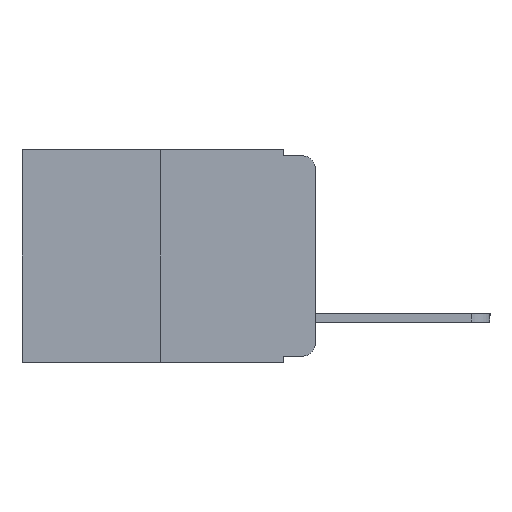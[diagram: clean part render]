
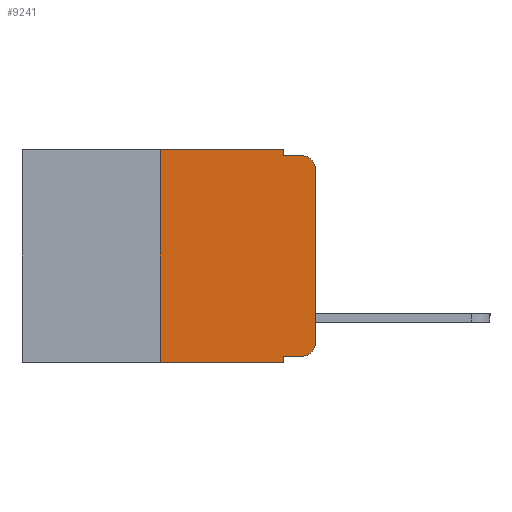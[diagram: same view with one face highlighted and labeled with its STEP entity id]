
A CAD part, left-side view. The second image highlights one B-rep face of the part: STEP entity #9241.
In plain terms, the highlighted planar face has unit normal (-1, 0, 0).
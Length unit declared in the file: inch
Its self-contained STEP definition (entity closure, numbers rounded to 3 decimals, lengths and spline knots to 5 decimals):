
#262 = LINE ( 'NONE', #21663, #22019 ) ;
#477 = CARTESIAN_POINT ( 'NONE',  ( 0., 0., -0.313 ) ) ;
#1154 = DIRECTION ( 'NONE',  ( 0., -1., 0. ) ) ;
#1220 = ORIENTED_EDGE ( 'NONE', *, *, #9397, .T. ) ;
#1235 = AXIS2_PLACEMENT_3D ( 'NONE', #17541, #7391, #19065 ) ;
#1457 = LINE ( 'NONE', #2063, #2033 ) ;
#1526 = VECTOR ( 'NONE', #12954, 39.37008 ) ;
#2030 = VECTOR ( 'NONE', #1154, 39.37008 ) ;
#2033 = VECTOR ( 'NONE', #12986, 39.37008 ) ;
#2063 = CARTESIAN_POINT ( 'NONE',  ( 0., 0.473, -0.343 ) ) ;
#2291 = CARTESIAN_POINT ( 'NONE',  ( 0., 0.051, 0. ) ) ;
#2404 = ORIENTED_EDGE ( 'NONE', *, *, #4663, .F. ) ;
#2716 = LINE ( 'NONE', #5729, #1526 ) ;
#2755 = VERTEX_POINT ( 'NONE', #20034 ) ;
#2882 = CARTESIAN_POINT ( 'NONE',  ( 0., 0.051, -0.343 ) ) ;
#3092 = DIRECTION ( 'NONE',  ( 0., 0., -1. ) ) ;
#3281 = VERTEX_POINT ( 'NONE', #19433 ) ;
#3611 = ORIENTED_EDGE ( 'NONE', *, *, #22121, .F. ) ;
#3684 = DIRECTION ( 'NONE',  ( -1., 0., 0. ) ) ;
#4008 = CARTESIAN_POINT ( 'NONE',  ( 0., 0.051, -0.333 ) ) ;
#4189 = ORIENTED_EDGE ( 'NONE', *, *, #5977, .T. ) ;
#4587 = CARTESIAN_POINT ( 'NONE',  ( 0., 0.02, -0.01 ) ) ;
#4663 = EDGE_CURVE ( 'NONE', #3281, #2755, #6049, .T. ) ;
#5001 = VERTEX_POINT ( 'NONE', #4008 ) ;
#5729 = CARTESIAN_POINT ( 'NONE',  ( 0., 0.051, -0.01 ) ) ;
#5977 = EDGE_CURVE ( 'NONE', #5001, #19971, #21554, .T. ) ;
#6049 = LINE ( 'NONE', #2291, #13855 ) ;
#6156 = CIRCLE ( 'NONE', #13313, 0.02 ) ;
#6426 = EDGE_CURVE ( 'NONE', #16449, #3281, #11781, .T. ) ;
#6481 = VERTEX_POINT ( 'NONE', #22135 ) ;
#6624 = DIRECTION ( 'NONE',  ( 0., -1., 0. ) ) ;
#6761 = CARTESIAN_POINT ( 'NONE',  ( 0., 0., -0.03 ) ) ;
#6831 = ORIENTED_EDGE ( 'NONE', *, *, #13273, .F. ) ;
#6907 = VECTOR ( 'NONE', #7201, 39.37008 ) ;
#7201 = DIRECTION ( 'NONE',  ( 0., 0., 1. ) ) ;
#7292 = EDGE_CURVE ( 'NONE', #6481, #16449, #10400, .T. ) ;
#7391 = DIRECTION ( 'NONE',  ( -1., 0., 0. ) ) ;
#7416 = ORIENTED_EDGE ( 'NONE', *, *, #6426, .F. ) ;
#8373 = VERTEX_POINT ( 'NONE', #2882 ) ;
#8388 = AXIS2_PLACEMENT_3D ( 'NONE', #12613, #19031, #9230 ) ;
#9230 = DIRECTION ( 'NONE',  ( 0., 0., -1. ) ) ;
#9241 = ADVANCED_FACE ( 'NONE', ( #13411 ), #14336, .F. ) ;
#9324 = EDGE_CURVE ( 'NONE', #6481, #8373, #1457, .T. ) ;
#9397 = EDGE_CURVE ( 'NONE', #9412, #12617, #18382, .T. ) ;
#9412 = VERTEX_POINT ( 'NONE', #477 ) ;
#9821 = CARTESIAN_POINT ( 'NONE',  ( 0., 0., 0. ) ) ;
#10215 = DIRECTION ( 'NONE',  ( 0., 0., -1. ) ) ;
#10400 = LINE ( 'NONE', #18922, #6907 ) ;
#11599 = VERTEX_POINT ( 'NONE', #4587 ) ;
#11781 = LINE ( 'NONE', #21665, #2030 ) ;
#12135 = ORIENTED_EDGE ( 'NONE', *, *, #7292, .F. ) ;
#12613 = CARTESIAN_POINT ( 'NONE',  ( 0., 0.473, 0. ) ) ;
#12617 = VERTEX_POINT ( 'NONE', #6761 ) ;
#12687 = ORIENTED_EDGE ( 'NONE', *, *, #9324, .T. ) ;
#12754 = CIRCLE ( 'NONE', #1235, 0.02 ) ;
#12954 = DIRECTION ( 'NONE',  ( 0., -1., 0. ) ) ;
#12986 = DIRECTION ( 'NONE',  ( 0., -1., 0. ) ) ;
#13184 = EDGE_LOOP ( 'NONE', ( #1220, #19649, #6831, #2404, #7416, #12135, #12687, #3611, #4189, #14291 ) ) ;
#13273 = EDGE_CURVE ( 'NONE', #2755, #11599, #2716, .T. ) ;
#13313 = AXIS2_PLACEMENT_3D ( 'NONE', #14408, #3684, #15995 ) ;
#13411 = FACE_OUTER_BOUND ( 'NONE', #13184, .T. ) ;
#13413 = CARTESIAN_POINT ( 'NONE',  ( 0., 0.25, 0. ) ) ;
#13855 = VECTOR ( 'NONE', #10215, 39.37008 ) ;
#14291 = ORIENTED_EDGE ( 'NONE', *, *, #21303, .T. ) ;
#14336 = PLANE ( 'NONE',  #8388 ) ;
#14408 = CARTESIAN_POINT ( 'NONE',  ( 0., 0.02, -0.313 ) ) ;
#15995 = DIRECTION ( 'NONE',  ( 0., 0., -1. ) ) ;
#16449 = VERTEX_POINT ( 'NONE', #13413 ) ;
#16971 = VECTOR ( 'NONE', #6624, 39.37008 ) ;
#17033 = EDGE_CURVE ( 'NONE', #12617, #11599, #12754, .T. ) ;
#17072 = CARTESIAN_POINT ( 'NONE',  ( 0., 0.02, -0.333 ) ) ;
#17541 = CARTESIAN_POINT ( 'NONE',  ( 0., 0.02, -0.03 ) ) ;
#18382 = LINE ( 'NONE', #9821, #21996 ) ;
#18922 = CARTESIAN_POINT ( 'NONE',  ( 0., 0.25, 0. ) ) ;
#19031 = DIRECTION ( 'NONE',  ( 1., 0., 0. ) ) ;
#19065 = DIRECTION ( 'NONE',  ( 0., 0., -1. ) ) ;
#19433 = CARTESIAN_POINT ( 'NONE',  ( 0., 0.051, 0. ) ) ;
#19649 = ORIENTED_EDGE ( 'NONE', *, *, #17033, .T. ) ;
#19971 = VERTEX_POINT ( 'NONE', #17072 ) ;
#20034 = CARTESIAN_POINT ( 'NONE',  ( 0., 0.051, -0.01 ) ) ;
#21117 = DIRECTION ( 'NONE',  ( 0., 0., 1. ) ) ;
#21303 = EDGE_CURVE ( 'NONE', #19971, #9412, #6156, .T. ) ;
#21462 = CARTESIAN_POINT ( 'NONE',  ( 0., 0.051, -0.333 ) ) ;
#21554 = LINE ( 'NONE', #21462, #16971 ) ;
#21663 = CARTESIAN_POINT ( 'NONE',  ( 0., 0.051, 0. ) ) ;
#21665 = CARTESIAN_POINT ( 'NONE',  ( 0., 0.473, 0. ) ) ;
#21996 = VECTOR ( 'NONE', #21117, 39.37008 ) ;
#22019 = VECTOR ( 'NONE', #3092, 39.37008 ) ;
#22121 = EDGE_CURVE ( 'NONE', #5001, #8373, #262, .T. ) ;
#22135 = CARTESIAN_POINT ( 'NONE',  ( 0., 0.25, -0.343 ) ) ;
